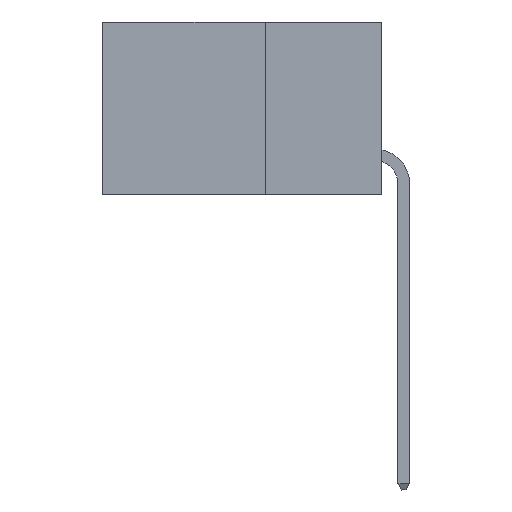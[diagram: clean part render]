
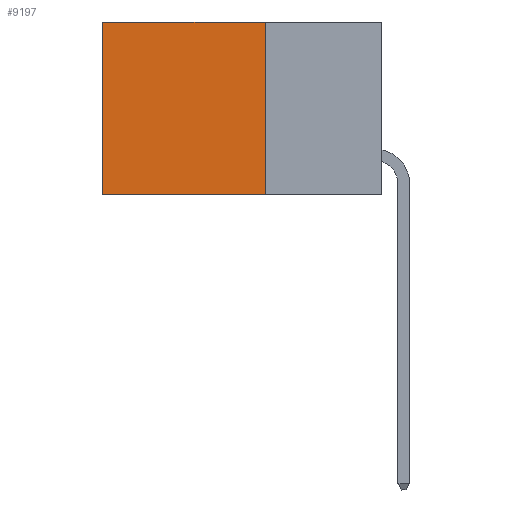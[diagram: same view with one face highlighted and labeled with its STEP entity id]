
A CAD part, left-side view. The second image highlights one B-rep face of the part: STEP entity #9197.
In plain terms, the highlighted planar face has unit normal (-1, 0, 0).
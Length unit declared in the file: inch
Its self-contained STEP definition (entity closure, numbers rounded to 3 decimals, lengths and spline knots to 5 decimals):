
#579 = ORIENTED_EDGE ( 'NONE', *, *, #10297, .F. ) ;
#723 = ORIENTED_EDGE ( 'NONE', *, *, #21623, .F. ) ;
#740 = VECTOR ( 'NONE', #6632, 39.37008 ) ;
#3509 = EDGE_CURVE ( 'NONE', #22798, #14807, #20880, .T. ) ;
#4749 = VECTOR ( 'NONE', #20140, 39.37008 ) ;
#5382 = VECTOR ( 'NONE', #15847, 39.37008 ) ;
#5661 = CARTESIAN_POINT ( 'NONE',  ( 0.2875, 0.6, -0.37 ) ) ;
#6024 = CARTESIAN_POINT ( 'NONE',  ( 0.2875, 0.6, 0. ) ) ;
#6541 = AXIS2_PLACEMENT_3D ( 'NONE', #14609, #6598, #20729 ) ;
#6598 = DIRECTION ( 'NONE',  ( 1., 0., 0. ) ) ;
#6632 = DIRECTION ( 'NONE',  ( 0., 0., -1. ) ) ;
#6948 = VECTOR ( 'NONE', #20486, 39.37008 ) ;
#7568 = LINE ( 'NONE', #12339, #6948 ) ;
#8524 = PLANE ( 'NONE',  #6541 ) ;
#8577 = EDGE_CURVE ( 'NONE', #14807, #21411, #11451, .T. ) ;
#8926 = ORIENTED_EDGE ( 'NONE', *, *, #3509, .T. ) ;
#9197 = ADVANCED_FACE ( 'NONE', ( #11728 ), #8524, .F. ) ;
#10297 = EDGE_CURVE ( 'NONE', #17626, #21411, #16698, .T. ) ;
#11451 = LINE ( 'NONE', #12604, #740 ) ;
#11508 = ORIENTED_EDGE ( 'NONE', *, *, #8577, .T. ) ;
#11728 = FACE_OUTER_BOUND ( 'NONE', #12356, .T. ) ;
#12339 = CARTESIAN_POINT ( 'NONE',  ( 0.2875, 0.25, 0. ) ) ;
#12356 = EDGE_LOOP ( 'NONE', ( #11508, #579, #723, #8926 ) ) ;
#12604 = CARTESIAN_POINT ( 'NONE',  ( 0.2875, 0.6, 0. ) ) ;
#14609 = CARTESIAN_POINT ( 'NONE',  ( 0.2875, 0.25, 0. ) ) ;
#14807 = VERTEX_POINT ( 'NONE', #6024 ) ;
#15847 = DIRECTION ( 'NONE',  ( 0., 1., 0. ) ) ;
#15941 = CARTESIAN_POINT ( 'NONE',  ( 0.2875, 0.25, -0.37 ) ) ;
#16698 = LINE ( 'NONE', #15941, #5382 ) ;
#17626 = VERTEX_POINT ( 'NONE', #20444 ) ;
#18071 = CARTESIAN_POINT ( 'NONE',  ( 0.2875, 0.25, 0. ) ) ;
#19780 = CARTESIAN_POINT ( 'NONE',  ( 0.2875, 0.25, 0. ) ) ;
#20140 = DIRECTION ( 'NONE',  ( 0., 1., 0. ) ) ;
#20444 = CARTESIAN_POINT ( 'NONE',  ( 0.2875, 0.25, -0.37 ) ) ;
#20486 = DIRECTION ( 'NONE',  ( 0., 0., -1. ) ) ;
#20729 = DIRECTION ( 'NONE',  ( 0., 0., -1. ) ) ;
#20880 = LINE ( 'NONE', #18071, #4749 ) ;
#21411 = VERTEX_POINT ( 'NONE', #5661 ) ;
#21623 = EDGE_CURVE ( 'NONE', #22798, #17626, #7568, .T. ) ;
#22798 = VERTEX_POINT ( 'NONE', #19780 ) ;
